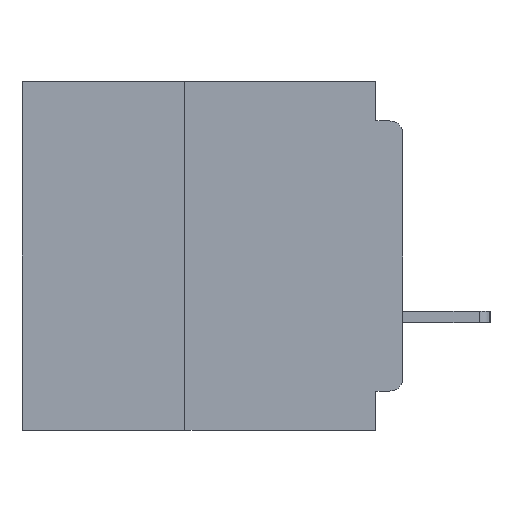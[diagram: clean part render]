
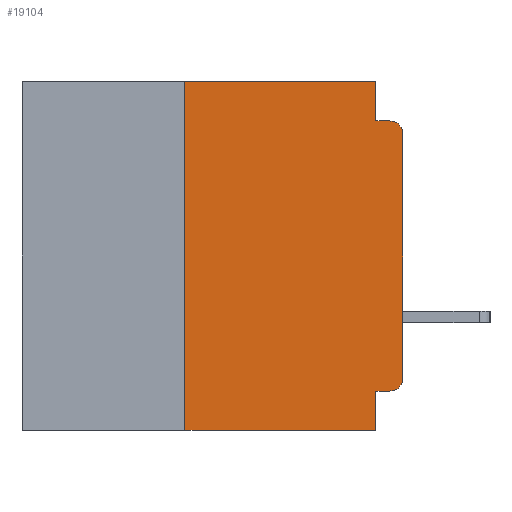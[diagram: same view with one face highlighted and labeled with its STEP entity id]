
A CAD part, left-side view. The second image highlights one B-rep face of the part: STEP entity #19104.
In plain terms, the highlighted planar face has unit normal (-1, 0, 0).
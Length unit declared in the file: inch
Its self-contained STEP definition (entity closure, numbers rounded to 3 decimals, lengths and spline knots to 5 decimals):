
#341 = CARTESIAN_POINT ( 'NONE',  ( 0., 0.031, 0. ) ) ;
#498 = CARTESIAN_POINT ( 'NONE',  ( 0., 0.015, -0.355 ) ) ;
#689 = CARTESIAN_POINT ( 'NONE',  ( 0., 0., -0.34 ) ) ;
#1372 = EDGE_CURVE ( 'NONE', #24664, #28872, #15685, .T. ) ;
#2994 = VERTEX_POINT ( 'NONE', #36126 ) ;
#3605 = DIRECTION ( 'NONE',  ( 0., -1., 0. ) ) ;
#4055 = EDGE_CURVE ( 'NONE', #19572, #2994, #14313, .T. ) ;
#4144 = DIRECTION ( 'NONE',  ( 1., 0., 0. ) ) ;
#4384 = VECTOR ( 'NONE', #5085, 39.37008 ) ;
#4954 = CIRCLE ( 'NONE', #23168, 0.015 ) ;
#4972 = CARTESIAN_POINT ( 'NONE',  ( 0., 0.437, 0. ) ) ;
#5063 = LINE ( 'NONE', #30990, #26588 ) ;
#5085 = DIRECTION ( 'NONE',  ( 0., -1., 0. ) ) ;
#5144 = DIRECTION ( 'NONE',  ( -1., 0., 0. ) ) ;
#6018 = ORIENTED_EDGE ( 'NONE', *, *, #18247, .F. ) ;
#6499 = CARTESIAN_POINT ( 'NONE',  ( 0., 0.015, -0.06 ) ) ;
#6579 = EDGE_CURVE ( 'NONE', #35350, #19572, #4954, .T. ) ;
#6712 = CARTESIAN_POINT ( 'NONE',  ( 0., 0.031, 0. ) ) ;
#7342 = LINE ( 'NONE', #17605, #20507 ) ;
#7689 = DIRECTION ( 'NONE',  ( 0., -1., 0. ) ) ;
#7715 = VECTOR ( 'NONE', #21494, 39.37008 ) ;
#8048 = CARTESIAN_POINT ( 'NONE',  ( 0., 0.25, 0. ) ) ;
#8940 = EDGE_CURVE ( 'NONE', #32056, #17626, #34790, .T. ) ;
#9319 = DIRECTION ( 'NONE',  ( 0., 0., -1. ) ) ;
#10425 = CARTESIAN_POINT ( 'NONE',  ( 0., 0.25, -0.4 ) ) ;
#10964 = CIRCLE ( 'NONE', #14052, 0.015 ) ;
#11401 = CARTESIAN_POINT ( 'NONE',  ( 0., 0.031, -0.045 ) ) ;
#11415 = VECTOR ( 'NONE', #7689, 39.37008 ) ;
#12988 = ORIENTED_EDGE ( 'NONE', *, *, #22663, .T. ) ;
#13219 = ORIENTED_EDGE ( 'NONE', *, *, #4055, .T. ) ;
#13245 = DIRECTION ( 'NONE',  ( 0., 0., 1. ) ) ;
#13712 = VECTOR ( 'NONE', #28576, 39.37008 ) ;
#14052 = AXIS2_PLACEMENT_3D ( 'NONE', #6499, #26165, #9319 ) ;
#14313 = LINE ( 'NONE', #18658, #7715 ) ;
#14805 = VECTOR ( 'NONE', #29338, 39.37008 ) ;
#15685 = LINE ( 'NONE', #6712, #14805 ) ;
#16120 = CARTESIAN_POINT ( 'NONE',  ( 0., 0.031, -0.355 ) ) ;
#17605 = CARTESIAN_POINT ( 'NONE',  ( 0., 0., -0.045 ) ) ;
#17626 = VERTEX_POINT ( 'NONE', #8048 ) ;
#18247 = EDGE_CURVE ( 'NONE', #33546, #18278, #5063, .T. ) ;
#18278 = VERTEX_POINT ( 'NONE', #25452 ) ;
#18658 = CARTESIAN_POINT ( 'NONE',  ( 0., 0., 0. ) ) ;
#18873 = LINE ( 'NONE', #33495, #11415 ) ;
#19104 = ADVANCED_FACE ( 'NONE', ( #26150 ), #29320, .F. ) ;
#19135 = ORIENTED_EDGE ( 'NONE', *, *, #36001, .F. ) ;
#19572 = VERTEX_POINT ( 'NONE', #689 ) ;
#19784 = DIRECTION ( 'NONE',  ( 0., 0., -1. ) ) ;
#20340 = CARTESIAN_POINT ( 'NONE',  ( 0., 0.015, -0.045 ) ) ;
#20507 = VECTOR ( 'NONE', #3605, 39.37008 ) ;
#20735 = CARTESIAN_POINT ( 'NONE',  ( 0., 0.25, -0.4 ) ) ;
#20947 = CARTESIAN_POINT ( 'NONE',  ( 0., 0.437, 0. ) ) ;
#21097 = ORIENTED_EDGE ( 'NONE', *, *, #8940, .F. ) ;
#21134 = AXIS2_PLACEMENT_3D ( 'NONE', #20947, #4144, #23789 ) ;
#21494 = DIRECTION ( 'NONE',  ( 0., 0., 1. ) ) ;
#21539 = EDGE_CURVE ( 'NONE', #35350, #33546, #28658, .T. ) ;
#21942 = CARTESIAN_POINT ( 'NONE',  ( 0., 0.015, -0.34 ) ) ;
#22663 = EDGE_CURVE ( 'NONE', #32056, #18278, #18873, .T. ) ;
#22900 = EDGE_LOOP ( 'NONE', ( #13219, #29945, #19135, #35969, #28620, #21097, #12988, #6018, #25759, #31599 ) ) ;
#23168 = AXIS2_PLACEMENT_3D ( 'NONE', #21942, #5144, #24786 ) ;
#23789 = DIRECTION ( 'NONE',  ( 0., 0., -1. ) ) ;
#24664 = VERTEX_POINT ( 'NONE', #341 ) ;
#24786 = DIRECTION ( 'NONE',  ( 0., 0., -1. ) ) ;
#25452 = CARTESIAN_POINT ( 'NONE',  ( 0., 0.031, -0.4 ) ) ;
#25744 = CARTESIAN_POINT ( 'NONE',  ( 0., 0., -0.355 ) ) ;
#25759 = ORIENTED_EDGE ( 'NONE', *, *, #21539, .F. ) ;
#26150 = FACE_OUTER_BOUND ( 'NONE', #22900, .T. ) ;
#26165 = DIRECTION ( 'NONE',  ( -1., 0., 0. ) ) ;
#26588 = VECTOR ( 'NONE', #19784, 39.37008 ) ;
#26793 = LINE ( 'NONE', #4972, #4384 ) ;
#28255 = VECTOR ( 'NONE', #13245, 39.37008 ) ;
#28576 = DIRECTION ( 'NONE',  ( 0., 1., 0. ) ) ;
#28620 = ORIENTED_EDGE ( 'NONE', *, *, #34503, .F. ) ;
#28658 = LINE ( 'NONE', #25744, #13712 ) ;
#28872 = VERTEX_POINT ( 'NONE', #11401 ) ;
#29320 = PLANE ( 'NONE',  #21134 ) ;
#29338 = DIRECTION ( 'NONE',  ( 0., 0., -1. ) ) ;
#29945 = ORIENTED_EDGE ( 'NONE', *, *, #33885, .T. ) ;
#30800 = VERTEX_POINT ( 'NONE', #20340 ) ;
#30990 = CARTESIAN_POINT ( 'NONE',  ( 0., 0.031, -0.4 ) ) ;
#31599 = ORIENTED_EDGE ( 'NONE', *, *, #6579, .T. ) ;
#32056 = VERTEX_POINT ( 'NONE', #20735 ) ;
#33495 = CARTESIAN_POINT ( 'NONE',  ( 0., 0.437, -0.4 ) ) ;
#33546 = VERTEX_POINT ( 'NONE', #16120 ) ;
#33885 = EDGE_CURVE ( 'NONE', #2994, #30800, #10964, .T. ) ;
#34503 = EDGE_CURVE ( 'NONE', #17626, #24664, #26793, .T. ) ;
#34790 = LINE ( 'NONE', #10425, #28255 ) ;
#35350 = VERTEX_POINT ( 'NONE', #498 ) ;
#35969 = ORIENTED_EDGE ( 'NONE', *, *, #1372, .F. ) ;
#36001 = EDGE_CURVE ( 'NONE', #28872, #30800, #7342, .T. ) ;
#36126 = CARTESIAN_POINT ( 'NONE',  ( 0., 0., -0.06 ) ) ;
